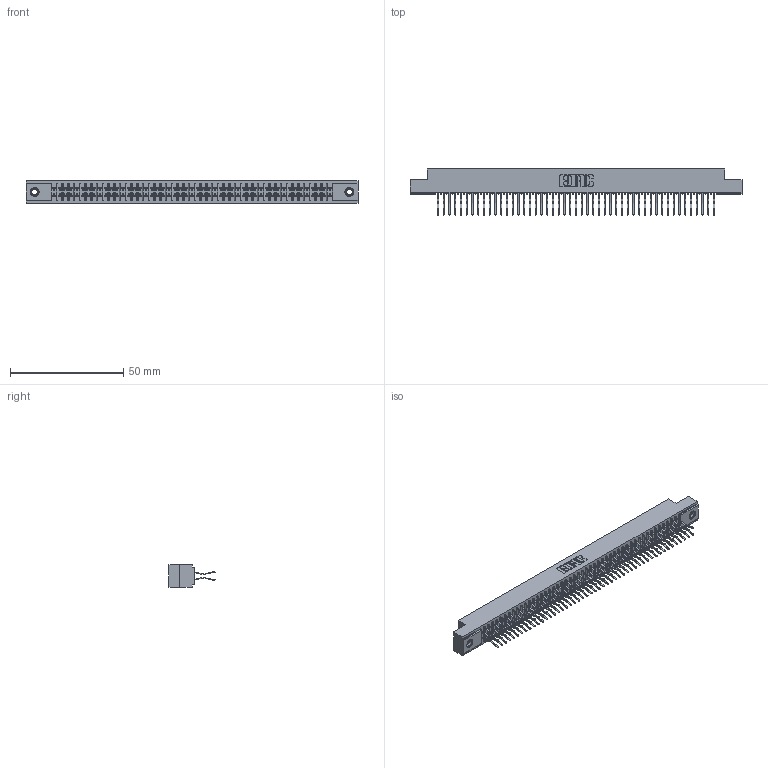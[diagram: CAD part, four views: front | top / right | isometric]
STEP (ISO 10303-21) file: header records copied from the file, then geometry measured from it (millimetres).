
FILE_DESCRIPTION (( 'STEP AP203' ), '1' );
FILE_NAME ('341-098-560-207.STEP', '2018-08-08T02:32:05', ( '' ), ( '' ), 'SwSTEP 2.0', 'SolidWorks 2016', '' );
FILE_SCHEMA (( 'CONFIG_CONTROL_DESIGN' ));
Length unit declared in the file: inch
Products named in the file (4): 341 Part_.156 (3.96) Dia Mounting Holes; 341-292-001_341-292-160; 345-250-001_345-250-005-103; 341-098-560-207
Assembly tree (101 placements, depth 2):
  341-098-560-207
    341 Part_.156 (3.96) Dia Mounting Holes
    341-292-001_341-292-160  x98
    345-250-001_345-250-005-103  x2
Bounding box: 146.69 x 20.37 x 10.16 mm (x, y, z)
Volume: 10921.9 mm3; surface area: 20369.4 mm2
Topology: 101 solids, 101 shells, 7036 faces, 20395 edges, 13226 vertices
Faces by surface type: plane 4020, cylinder 2804, sphere 100, torus 100, cone 12
Entity records: 59693 total; most frequent: CARTESIAN_POINT 9906, ORIENTED_EDGE 9838, DIRECTION 9623, EDGE_CURVE 4919, LINE 3973, VECTOR 3973, VERTEX_POINT 3108, AXIS2_PLACEMENT_3D 2825
